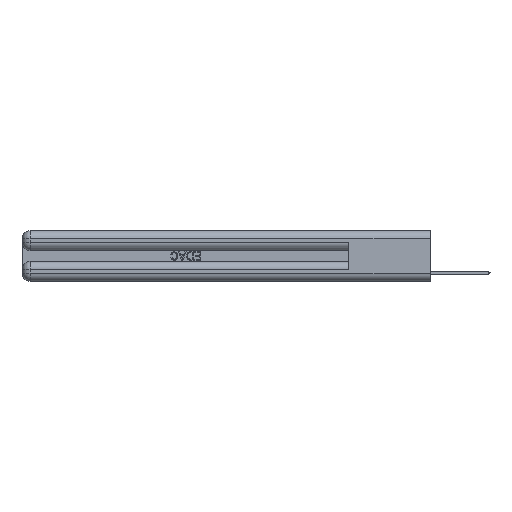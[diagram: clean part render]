
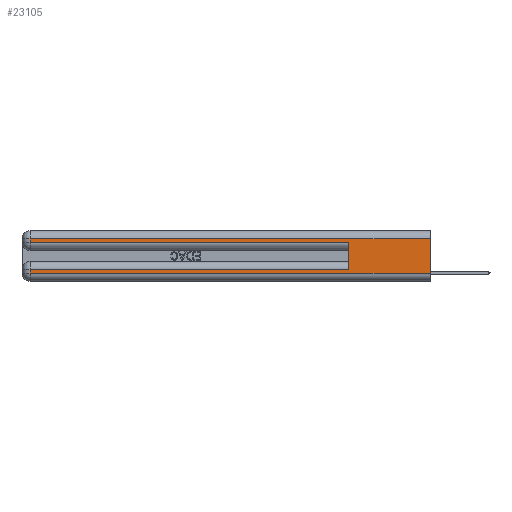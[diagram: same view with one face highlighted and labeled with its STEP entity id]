
A CAD part, left-side view. The second image highlights one B-rep face of the part: STEP entity #23105.
In plain terms, the highlighted planar face has unit normal (-1, 0, 0).
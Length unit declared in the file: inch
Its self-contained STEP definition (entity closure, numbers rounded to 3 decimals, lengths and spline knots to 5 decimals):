
#230 = VERTEX_POINT ( 'NONE', #24296 ) ;
#316 = VECTOR ( 'NONE', #25853, 39.37008 ) ;
#1099 = ORIENTED_EDGE ( 'NONE', *, *, #8303, .F. ) ;
#1558 = EDGE_CURVE ( 'NONE', #9878, #18294, #24418, .T. ) ;
#1702 = VERTEX_POINT ( 'NONE', #6934 ) ;
#2571 = VECTOR ( 'NONE', #12816, 39.37008 ) ;
#2903 = DIRECTION ( 'NONE',  ( 0., 0., -1. ) ) ;
#3426 = EDGE_CURVE ( 'NONE', #230, #8762, #13629, .T. ) ;
#3819 = ORIENTED_EDGE ( 'NONE', *, *, #4452, .T. ) ;
#4093 = ORIENTED_EDGE ( 'NONE', *, *, #1558, .F. ) ;
#4110 = PLANE ( 'NONE',  #21621 ) ;
#4452 = EDGE_CURVE ( 'NONE', #9878, #23710, #13909, .T. ) ;
#4596 = VERTEX_POINT ( 'NONE', #15755 ) ;
#4879 = ORIENTED_EDGE ( 'NONE', *, *, #20353, .T. ) ;
#5279 = FACE_OUTER_BOUND ( 'NONE', #15677, .T. ) ;
#6271 = CARTESIAN_POINT ( 'NONE',  ( 0., 2.94, 0.085 ) ) ;
#6649 = CARTESIAN_POINT ( 'NONE',  ( 0., 2.94, 0.285 ) ) ;
#6934 = CARTESIAN_POINT ( 'NONE',  ( 0., 0., 0.31 ) ) ;
#7028 = CARTESIAN_POINT ( 'NONE',  ( 0., 0., 0.085 ) ) ;
#7299 = DIRECTION ( 'NONE',  ( 0., 0., -1. ) ) ;
#7691 = CARTESIAN_POINT ( 'NONE',  ( 0., 0.6, 0.285 ) ) ;
#8303 = EDGE_CURVE ( 'NONE', #1702, #17349, #16057, .T. ) ;
#8326 = VECTOR ( 'NONE', #18584, 39.37008 ) ;
#8762 = VERTEX_POINT ( 'NONE', #6649 ) ;
#9878 = VERTEX_POINT ( 'NONE', #14136 ) ;
#10715 = CARTESIAN_POINT ( 'NONE',  ( 0., 2.94, 0.37 ) ) ;
#10766 = VECTOR ( 'NONE', #12960, 39.37008 ) ;
#11445 = DIRECTION ( 'NONE',  ( 0., 1., 0. ) ) ;
#12195 = DIRECTION ( 'NONE',  ( 1., 0., 0. ) ) ;
#12281 = ORIENTED_EDGE ( 'NONE', *, *, #3426, .T. ) ;
#12342 = LINE ( 'NONE', #21639, #15273 ) ;
#12816 = DIRECTION ( 'NONE',  ( 0., 0., -1. ) ) ;
#12960 = DIRECTION ( 'NONE',  ( 0., 1., 0. ) ) ;
#13129 = EDGE_CURVE ( 'NONE', #8762, #18294, #21130, .T. ) ;
#13629 = LINE ( 'NONE', #10715, #2571 ) ;
#13909 = LINE ( 'NONE', #7028, #24308 ) ;
#14136 = CARTESIAN_POINT ( 'NONE',  ( 0., 0.6, 0.085 ) ) ;
#14287 = DIRECTION ( 'NONE',  ( 0., 0., -1. ) ) ;
#14984 = CARTESIAN_POINT ( 'NONE',  ( 0., 0., 0.31 ) ) ;
#15188 = ORIENTED_EDGE ( 'NONE', *, *, #21660, .T. ) ;
#15273 = VECTOR ( 'NONE', #2903, 39.37008 ) ;
#15677 = EDGE_LOOP ( 'NONE', ( #1099, #4879, #12281, #18597, #4093, #3819, #15188, #18055 ) ) ;
#15755 = CARTESIAN_POINT ( 'NONE',  ( 0., 2.94, 0.06 ) ) ;
#16057 = LINE ( 'NONE', #26071, #17661 ) ;
#17154 = CARTESIAN_POINT ( 'NONE',  ( 0., 0., 0.285 ) ) ;
#17349 = VERTEX_POINT ( 'NONE', #18736 ) ;
#17661 = VECTOR ( 'NONE', #7299, 39.37008 ) ;
#18055 = ORIENTED_EDGE ( 'NONE', *, *, #18442, .T. ) ;
#18294 = VERTEX_POINT ( 'NONE', #7691 ) ;
#18393 = CARTESIAN_POINT ( 'NONE',  ( 0., 0., 0.37 ) ) ;
#18442 = EDGE_CURVE ( 'NONE', #4596, #17349, #19373, .T. ) ;
#18494 = CARTESIAN_POINT ( 'NONE',  ( 0., 0., 0.06 ) ) ;
#18584 = DIRECTION ( 'NONE',  ( 0., -1., 0. ) ) ;
#18597 = ORIENTED_EDGE ( 'NONE', *, *, #13129, .T. ) ;
#18736 = CARTESIAN_POINT ( 'NONE',  ( 0., 0., 0.06 ) ) ;
#19373 = LINE ( 'NONE', #18494, #8326 ) ;
#20353 = EDGE_CURVE ( 'NONE', #1702, #230, #24419, .T. ) ;
#20547 = VECTOR ( 'NONE', #26704, 39.37008 ) ;
#21130 = LINE ( 'NONE', #17154, #316 ) ;
#21621 = AXIS2_PLACEMENT_3D ( 'NONE', #18393, #12195, #14287 ) ;
#21639 = CARTESIAN_POINT ( 'NONE',  ( 0., 2.94, 0.37 ) ) ;
#21660 = EDGE_CURVE ( 'NONE', #23710, #4596, #12342, .T. ) ;
#23105 = ADVANCED_FACE ( 'NONE', ( #5279 ), #4110, .F. ) ;
#23168 = CARTESIAN_POINT ( 'NONE',  ( 0., 0.6, 0.145 ) ) ;
#23710 = VERTEX_POINT ( 'NONE', #6271 ) ;
#24296 = CARTESIAN_POINT ( 'NONE',  ( 0., 2.94, 0.31 ) ) ;
#24308 = VECTOR ( 'NONE', #11445, 39.37008 ) ;
#24418 = LINE ( 'NONE', #23168, #20547 ) ;
#24419 = LINE ( 'NONE', #14984, #10766 ) ;
#25853 = DIRECTION ( 'NONE',  ( 0., -1., 0. ) ) ;
#26071 = CARTESIAN_POINT ( 'NONE',  ( 0., 0., 0.37 ) ) ;
#26704 = DIRECTION ( 'NONE',  ( 0., 0., 1. ) ) ;
